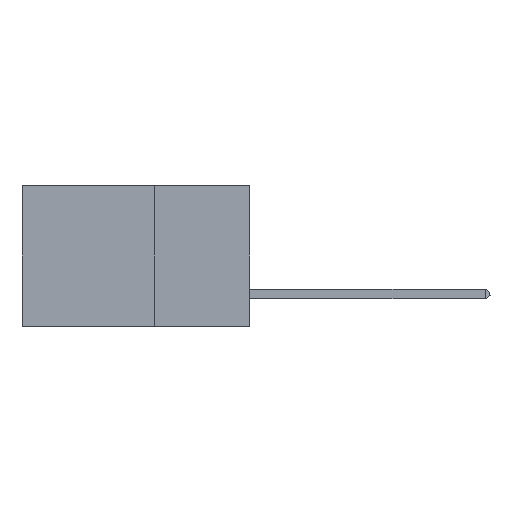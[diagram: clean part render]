
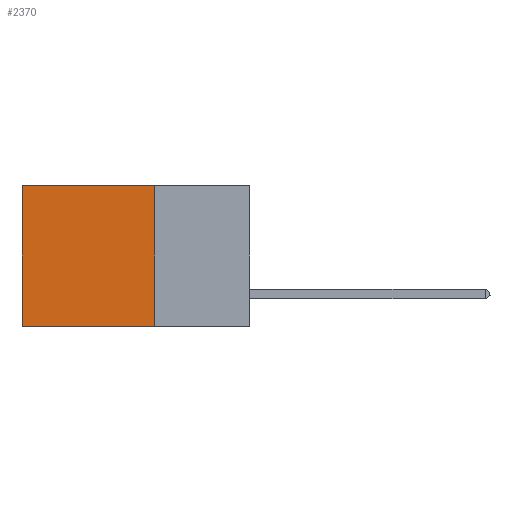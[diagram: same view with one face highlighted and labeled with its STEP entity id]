
A CAD part, left-side view. The second image highlights one B-rep face of the part: STEP entity #2370.
In plain terms, the highlighted planar face has unit normal (-1, 0, 0).
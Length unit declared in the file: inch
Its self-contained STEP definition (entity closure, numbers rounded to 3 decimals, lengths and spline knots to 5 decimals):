
#325 = DIRECTION ( 'NONE',  ( 1., 0., 0. ) ) ;
#416 = DIRECTION ( 'NONE',  ( 0., 1., 0. ) ) ;
#1132 = CARTESIAN_POINT ( 'NONE',  ( 0.2875, 0.6, -0.37 ) ) ;
#1225 = EDGE_LOOP ( 'NONE', ( #15193, #14473, #10928, #10217 ) ) ;
#1226 = EDGE_CURVE ( 'NONE', #3956, #4623, #11982, .T. ) ;
#2319 = PLANE ( 'NONE',  #11857 ) ;
#2370 = ADVANCED_FACE ( 'NONE', ( #5158 ), #2319, .F. ) ;
#2398 = VECTOR ( 'NONE', #8895, 39.37008 ) ;
#2413 = VERTEX_POINT ( 'NONE', #15537 ) ;
#2827 = CARTESIAN_POINT ( 'NONE',  ( 0.2875, 0.25, 0. ) ) ;
#3956 = VERTEX_POINT ( 'NONE', #7062 ) ;
#4196 = LINE ( 'NONE', #9253, #9438 ) ;
#4603 = CARTESIAN_POINT ( 'NONE',  ( 0.2875, 0.25, -0.37 ) ) ;
#4623 = VERTEX_POINT ( 'NONE', #4603 ) ;
#5158 = FACE_OUTER_BOUND ( 'NONE', #1225, .T. ) ;
#5730 = DIRECTION ( 'NONE',  ( 0., 1., 0. ) ) ;
#5855 = EDGE_CURVE ( 'NONE', #2413, #9290, #12010, .T. ) ;
#6339 = CARTESIAN_POINT ( 'NONE',  ( 0.2875, 0.25, 0. ) ) ;
#7012 = EDGE_CURVE ( 'NONE', #4623, #9290, #10814, .T. ) ;
#7062 = CARTESIAN_POINT ( 'NONE',  ( 0.2875, 0.25, 0. ) ) ;
#8457 = CARTESIAN_POINT ( 'NONE',  ( 0.2875, 0.6, 0. ) ) ;
#8895 = DIRECTION ( 'NONE',  ( 0., 0., -1. ) ) ;
#9245 = EDGE_CURVE ( 'NONE', #3956, #2413, #4196, .T. ) ;
#9253 = CARTESIAN_POINT ( 'NONE',  ( 0.2875, 0.25, 0. ) ) ;
#9290 = VERTEX_POINT ( 'NONE', #1132 ) ;
#9438 = VECTOR ( 'NONE', #5730, 39.37008 ) ;
#10217 = ORIENTED_EDGE ( 'NONE', *, *, #9245, .T. ) ;
#10624 = VECTOR ( 'NONE', #416, 39.37008 ) ;
#10814 = LINE ( 'NONE', #14787, #10624 ) ;
#10928 = ORIENTED_EDGE ( 'NONE', *, *, #1226, .F. ) ;
#11071 = DIRECTION ( 'NONE',  ( 0., 0., -1. ) ) ;
#11857 = AXIS2_PLACEMENT_3D ( 'NONE', #6339, #325, #11071 ) ;
#11982 = LINE ( 'NONE', #2827, #2398 ) ;
#12010 = LINE ( 'NONE', #8457, #14053 ) ;
#14053 = VECTOR ( 'NONE', #15556, 39.37008 ) ;
#14473 = ORIENTED_EDGE ( 'NONE', *, *, #7012, .F. ) ;
#14787 = CARTESIAN_POINT ( 'NONE',  ( 0.2875, 0.25, -0.37 ) ) ;
#15193 = ORIENTED_EDGE ( 'NONE', *, *, #5855, .T. ) ;
#15537 = CARTESIAN_POINT ( 'NONE',  ( 0.2875, 0.6, 0. ) ) ;
#15556 = DIRECTION ( 'NONE',  ( 0., 0., -1. ) ) ;
